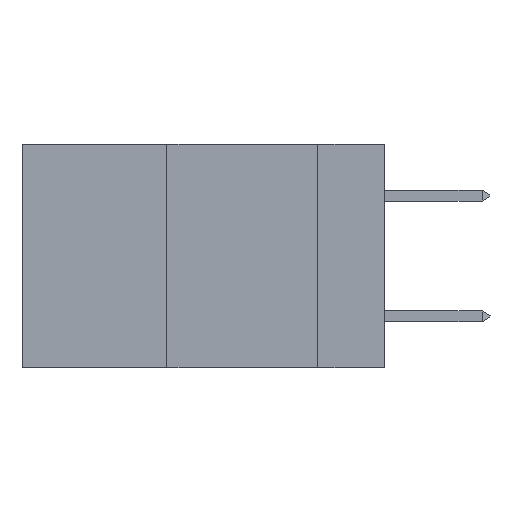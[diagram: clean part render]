
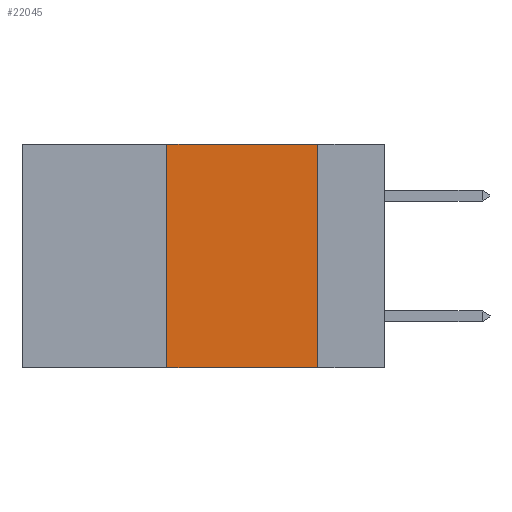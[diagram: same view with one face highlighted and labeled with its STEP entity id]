
A CAD part, left-side view. The second image highlights one B-rep face of the part: STEP entity #22045.
In plain terms, the highlighted planar face has unit normal (-1, 0, 0).
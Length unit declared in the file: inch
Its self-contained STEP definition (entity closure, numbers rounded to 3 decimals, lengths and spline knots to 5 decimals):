
#1239 = VERTEX_POINT ( 'NONE', #9851 ) ;
#3081 = CARTESIAN_POINT ( 'NONE',  ( 0., 0.6, 0. ) ) ;
#5157 = EDGE_CURVE ( 'NONE', #14841, #1239, #13500, .T. ) ;
#6022 = AXIS2_PLACEMENT_3D ( 'NONE', #30729, #27980, #6316 ) ;
#6316 = DIRECTION ( 'NONE',  ( 0., 0., -1. ) ) ;
#7015 = VERTEX_POINT ( 'NONE', #36208 ) ;
#7071 = CARTESIAN_POINT ( 'NONE',  ( 0., 0.11, 0. ) ) ;
#7631 = DIRECTION ( 'NONE',  ( 0., 0., -1. ) ) ;
#9851 = CARTESIAN_POINT ( 'NONE',  ( 0., 0.11, 0. ) ) ;
#11092 = CARTESIAN_POINT ( 'NONE',  ( 0., 0.6, -0.37 ) ) ;
#11878 = ORIENTED_EDGE ( 'NONE', *, *, #23689, .T. ) ;
#13500 = LINE ( 'NONE', #3081, #14215 ) ;
#14215 = VECTOR ( 'NONE', #14297, 39.37008 ) ;
#14231 = EDGE_LOOP ( 'NONE', ( #15259, #31933, #26361, #11878 ) ) ;
#14297 = DIRECTION ( 'NONE',  ( 0., -1., 0. ) ) ;
#14841 = VERTEX_POINT ( 'NONE', #26065 ) ;
#15259 = ORIENTED_EDGE ( 'NONE', *, *, #19959, .F. ) ;
#16166 = CARTESIAN_POINT ( 'NONE',  ( 0., 0.11, -0.37 ) ) ;
#19905 = LINE ( 'NONE', #11092, #27196 ) ;
#19959 = EDGE_CURVE ( 'NONE', #1239, #33418, #21423, .T. ) ;
#20996 = VECTOR ( 'NONE', #21238, 39.37008 ) ;
#21238 = DIRECTION ( 'NONE',  ( 0., 0., 1. ) ) ;
#21421 = CARTESIAN_POINT ( 'NONE',  ( 0., 0.36, 0. ) ) ;
#21423 = LINE ( 'NONE', #7071, #23046 ) ;
#22045 = ADVANCED_FACE ( 'NONE', ( #33468 ), #33293, .F. ) ;
#22490 = DIRECTION ( 'NONE',  ( 0., -1., 0. ) ) ;
#23046 = VECTOR ( 'NONE', #7631, 39.37008 ) ;
#23689 = EDGE_CURVE ( 'NONE', #7015, #33418, #19905, .T. ) ;
#26065 = CARTESIAN_POINT ( 'NONE',  ( 0., 0.36, 0. ) ) ;
#26361 = ORIENTED_EDGE ( 'NONE', *, *, #35540, .F. ) ;
#26878 = LINE ( 'NONE', #21421, #20996 ) ;
#27196 = VECTOR ( 'NONE', #22490, 39.37008 ) ;
#27980 = DIRECTION ( 'NONE',  ( 1., 0., 0. ) ) ;
#30729 = CARTESIAN_POINT ( 'NONE',  ( 0., 0.6, 0. ) ) ;
#31933 = ORIENTED_EDGE ( 'NONE', *, *, #5157, .F. ) ;
#33293 = PLANE ( 'NONE',  #6022 ) ;
#33418 = VERTEX_POINT ( 'NONE', #16166 ) ;
#33468 = FACE_OUTER_BOUND ( 'NONE', #14231, .T. ) ;
#35540 = EDGE_CURVE ( 'NONE', #7015, #14841, #26878, .T. ) ;
#36208 = CARTESIAN_POINT ( 'NONE',  ( 0., 0.36, -0.37 ) ) ;
